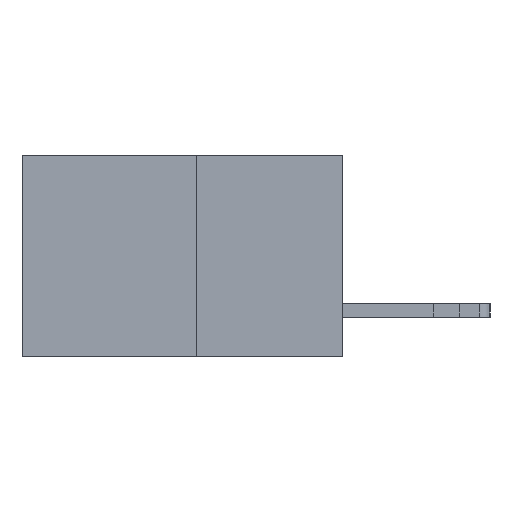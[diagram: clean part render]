
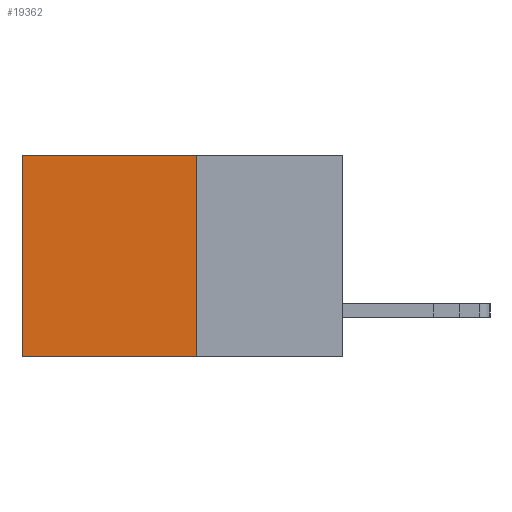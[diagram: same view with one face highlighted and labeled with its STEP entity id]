
A CAD part, left-side view. The second image highlights one B-rep face of the part: STEP entity #19362.
In plain terms, the highlighted planar face has unit normal (-1, 0, 0).
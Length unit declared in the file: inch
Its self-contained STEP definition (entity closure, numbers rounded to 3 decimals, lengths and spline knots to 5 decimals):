
#1845 = EDGE_CURVE ( 'NONE', #18715, #17791, #20360, .T. ) ;
#2722 = CARTESIAN_POINT ( 'NONE',  ( 0.277, 0.27, -0.37 ) ) ;
#3088 = VERTEX_POINT ( 'NONE', #19321 ) ;
#4096 = EDGE_CURVE ( 'NONE', #17791, #3088, #19218, .T. ) ;
#4437 = DIRECTION ( 'NONE',  ( 0., 0., -1. ) ) ;
#5612 = ORIENTED_EDGE ( 'NONE', *, *, #8909, .F. ) ;
#5777 = VERTEX_POINT ( 'NONE', #10365 ) ;
#6095 = CARTESIAN_POINT ( 'NONE',  ( 0.277, 0.59, -0.37 ) ) ;
#6350 = ORIENTED_EDGE ( 'NONE', *, *, #15966, .F. ) ;
#6537 = DIRECTION ( 'NONE',  ( 0., 0., -1. ) ) ;
#6565 = DIRECTION ( 'NONE',  ( 0., 0., -1. ) ) ;
#7901 = FACE_OUTER_BOUND ( 'NONE', #8050, .T. ) ;
#8050 = EDGE_LOOP ( 'NONE', ( #14379, #5612, #6350, #15886 ) ) ;
#8503 = CARTESIAN_POINT ( 'NONE',  ( 0.277, 0.27, 0. ) ) ;
#8909 = EDGE_CURVE ( 'NONE', #5777, #3088, #20409, .T. ) ;
#9646 = VECTOR ( 'NONE', #4437, 39.37008 ) ;
#9744 = CARTESIAN_POINT ( 'NONE',  ( 0.277, 0.27, -0.37 ) ) ;
#10365 = CARTESIAN_POINT ( 'NONE',  ( 0.277, 0.27, -0.37 ) ) ;
#10423 = VECTOR ( 'NONE', #6537, 39.37008 ) ;
#12102 = VECTOR ( 'NONE', #13537, 39.37008 ) ;
#12160 = VECTOR ( 'NONE', #21307, 39.37008 ) ;
#12496 = CARTESIAN_POINT ( 'NONE',  ( 0.277, 0.59, 0. ) ) ;
#12961 = AXIS2_PLACEMENT_3D ( 'NONE', #14869, #16535, #6565 ) ;
#13233 = PLANE ( 'NONE',  #12961 ) ;
#13537 = DIRECTION ( 'NONE',  ( 0., 1., 0. ) ) ;
#14086 = LINE ( 'NONE', #2722, #9646 ) ;
#14379 = ORIENTED_EDGE ( 'NONE', *, *, #4096, .T. ) ;
#14869 = CARTESIAN_POINT ( 'NONE',  ( 0.277, 0.27, -0.37 ) ) ;
#15886 = ORIENTED_EDGE ( 'NONE', *, *, #1845, .T. ) ;
#15966 = EDGE_CURVE ( 'NONE', #18715, #5777, #14086, .T. ) ;
#16535 = DIRECTION ( 'NONE',  ( 1., 0., 0. ) ) ;
#17791 = VERTEX_POINT ( 'NONE', #12496 ) ;
#18214 = CARTESIAN_POINT ( 'NONE',  ( 0.277, 0.27, 0. ) ) ;
#18715 = VERTEX_POINT ( 'NONE', #18214 ) ;
#19218 = LINE ( 'NONE', #6095, #10423 ) ;
#19321 = CARTESIAN_POINT ( 'NONE',  ( 0.277, 0.59, -0.37 ) ) ;
#19362 = ADVANCED_FACE ( 'NONE', ( #7901 ), #13233, .F. ) ;
#20360 = LINE ( 'NONE', #8503, #12102 ) ;
#20409 = LINE ( 'NONE', #9744, #12160 ) ;
#21307 = DIRECTION ( 'NONE',  ( 0., 1., 0. ) ) ;
